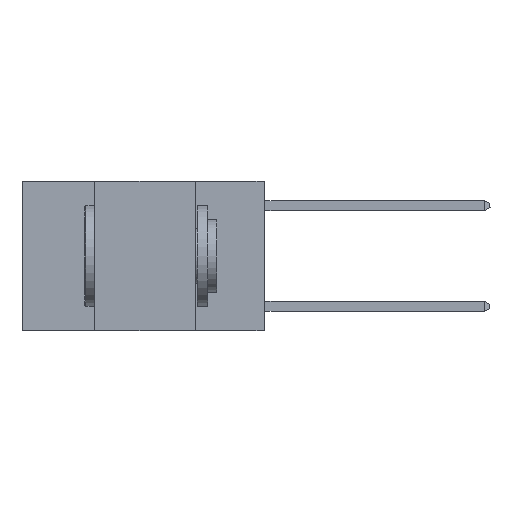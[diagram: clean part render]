
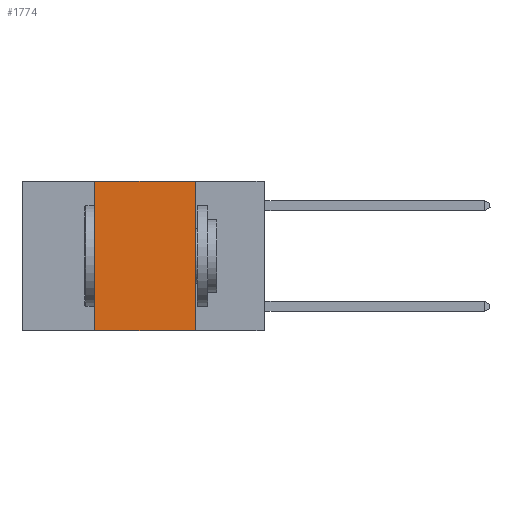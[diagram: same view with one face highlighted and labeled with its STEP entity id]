
A CAD part, left-side view. The second image highlights one B-rep face of the part: STEP entity #1774.
In plain terms, the highlighted planar face has unit normal (-1, 0, 0).
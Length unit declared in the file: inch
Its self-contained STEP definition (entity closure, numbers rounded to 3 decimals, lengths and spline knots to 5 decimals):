
#340 = VERTEX_POINT ( 'NONE', #4257 ) ;
#739 = VECTOR ( 'NONE', #2640, 39.37008 ) ;
#1060 = LINE ( 'NONE', #7052, #7343 ) ;
#1092 = EDGE_CURVE ( 'NONE', #340, #5705, #2802, .T. ) ;
#1268 = CARTESIAN_POINT ( 'NONE',  ( 0., 0.42, 0. ) ) ;
#1532 = ORIENTED_EDGE ( 'NONE', *, *, #6371, .F. ) ;
#1588 = CARTESIAN_POINT ( 'NONE',  ( 0., 0.42, 0. ) ) ;
#1774 = ADVANCED_FACE ( 'NONE', ( #2136 ), #7342, .F. ) ;
#1817 = VECTOR ( 'NONE', #8397, 39.37008 ) ;
#1891 = ORIENTED_EDGE ( 'NONE', *, *, #6454, .F. ) ;
#2065 = CARTESIAN_POINT ( 'NONE',  ( 0., 0.17, 0. ) ) ;
#2136 = FACE_OUTER_BOUND ( 'NONE', #2483, .T. ) ;
#2315 = ORIENTED_EDGE ( 'NONE', *, *, #8653, .T. ) ;
#2483 = EDGE_LOOP ( 'NONE', ( #1532, #1891, #5263, #2315 ) ) ;
#2640 = DIRECTION ( 'NONE',  ( 0., 0., 1. ) ) ;
#2802 = LINE ( 'NONE', #1268, #739 ) ;
#3072 = DIRECTION ( 'NONE',  ( 0., -1., 0. ) ) ;
#3448 = VECTOR ( 'NONE', #7717, 39.37008 ) ;
#3793 = VERTEX_POINT ( 'NONE', #2065 ) ;
#4257 = CARTESIAN_POINT ( 'NONE',  ( 0., 0.42, -0.37 ) ) ;
#4288 = AXIS2_PLACEMENT_3D ( 'NONE', #7270, #7193, #7070 ) ;
#5263 = ORIENTED_EDGE ( 'NONE', *, *, #1092, .F. ) ;
#5705 = VERTEX_POINT ( 'NONE', #1588 ) ;
#6177 = CARTESIAN_POINT ( 'NONE',  ( 0., 0.17, 0. ) ) ;
#6371 = EDGE_CURVE ( 'NONE', #3793, #6382, #9682, .T. ) ;
#6382 = VERTEX_POINT ( 'NONE', #6990 ) ;
#6454 = EDGE_CURVE ( 'NONE', #5705, #3793, #1060, .T. ) ;
#6990 = CARTESIAN_POINT ( 'NONE',  ( 0., 0.17, -0.37 ) ) ;
#7052 = CARTESIAN_POINT ( 'NONE',  ( 0., 0.6, 0. ) ) ;
#7070 = DIRECTION ( 'NONE',  ( 0., 0., -1. ) ) ;
#7193 = DIRECTION ( 'NONE',  ( 1., 0., 0. ) ) ;
#7270 = CARTESIAN_POINT ( 'NONE',  ( 0., 0.6, 0. ) ) ;
#7342 = PLANE ( 'NONE',  #4288 ) ;
#7343 = VECTOR ( 'NONE', #3072, 39.37008 ) ;
#7717 = DIRECTION ( 'NONE',  ( 0., -1., 0. ) ) ;
#7858 = LINE ( 'NONE', #9874, #3448 ) ;
#8397 = DIRECTION ( 'NONE',  ( 0., 0., -1. ) ) ;
#8653 = EDGE_CURVE ( 'NONE', #340, #6382, #7858, .T. ) ;
#9682 = LINE ( 'NONE', #6177, #1817 ) ;
#9874 = CARTESIAN_POINT ( 'NONE',  ( 0., 0.6, -0.37 ) ) ;
